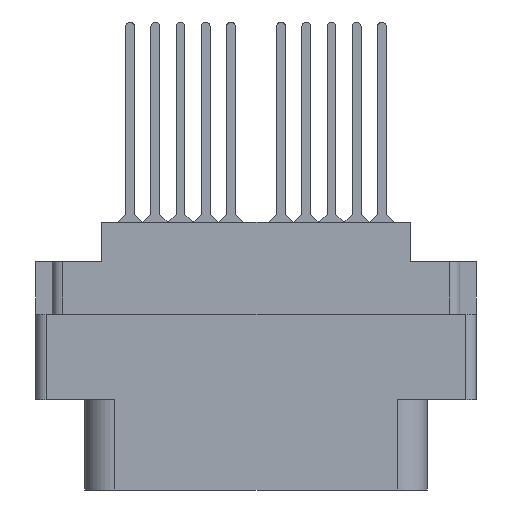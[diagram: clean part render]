
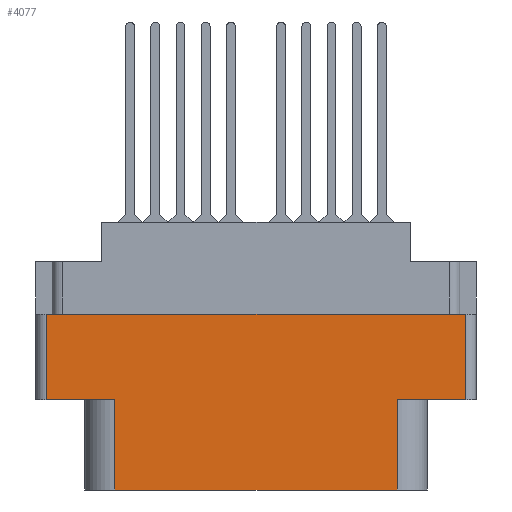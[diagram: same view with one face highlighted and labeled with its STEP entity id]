
A CAD part, front view. The second image highlights one B-rep face of the part: STEP entity #4077.
In plain terms, the highlighted planar face has unit normal (0, -1, 0).
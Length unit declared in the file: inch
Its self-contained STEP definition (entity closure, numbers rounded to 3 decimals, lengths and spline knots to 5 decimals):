
#502 = VECTOR ( 'NONE', #12374, 39.37008 ) ;
#558 = FACE_OUTER_BOUND ( 'NONE', #7926, .T. ) ;
#687 = VERTEX_POINT ( 'NONE', #7969 ) ;
#767 = CARTESIAN_POINT ( 'NONE',  ( -0.42052, -0.343, -0.798 ) ) ;
#2515 = VECTOR ( 'NONE', #4962, 39.37008 ) ;
#2782 = VERTEX_POINT ( 'NONE', #19760 ) ;
#3194 = ORIENTED_EDGE ( 'NONE', *, *, #14946, .T. ) ;
#4077 = ADVANCED_FACE ( 'NONE', ( #558 ), #27194, .T. ) ;
#4551 = VECTOR ( 'NONE', #13464, 39.37008 ) ;
#4962 = DIRECTION ( 'NONE',  ( 0., 0., -1. ) ) ;
#5088 = VECTOR ( 'NONE', #18477, 39.37008 ) ;
#5270 = DIRECTION ( 'NONE',  ( -1., 0., 0. ) ) ;
#5711 = CARTESIAN_POINT ( 'NONE',  ( 0.624, -0.343, -0.529 ) ) ;
#5946 = EDGE_CURVE ( 'NONE', #23747, #13217, #25041, .T. ) ;
#6018 = CARTESIAN_POINT ( 'NONE',  ( 0.624, -0.343, -0.274 ) ) ;
#6311 = ORIENTED_EDGE ( 'NONE', *, *, #12337, .T. ) ;
#6898 = CARTESIAN_POINT ( 'NONE',  ( -0.42052, -0.343, -0.529 ) ) ;
#7129 = LINE ( 'NONE', #11710, #5088 ) ;
#7200 = LINE ( 'NONE', #22389, #12022 ) ;
#7605 = AXIS2_PLACEMENT_3D ( 'NONE', #9855, #12155, #18536 ) ;
#7799 = ORIENTED_EDGE ( 'NONE', *, *, #14473, .F. ) ;
#7926 = EDGE_LOOP ( 'NONE', ( #25615, #3194, #23369, #15435, #6311, #18955, #7799, #14223 ) ) ;
#7969 = CARTESIAN_POINT ( 'NONE',  ( -0.42052, -0.343, -0.798 ) ) ;
#9855 = CARTESIAN_POINT ( 'NONE',  ( -0.656, -0.343, -0.798 ) ) ;
#10859 = DIRECTION ( 'NONE',  ( 0., 0., 1. ) ) ;
#11710 = CARTESIAN_POINT ( 'NONE',  ( 0., -0.343, -0.274 ) ) ;
#11861 = DIRECTION ( 'NONE',  ( 0., 0., -1. ) ) ;
#12022 = VECTOR ( 'NONE', #5270, 39.37008 ) ;
#12155 = DIRECTION ( 'NONE',  ( 0., -1., 0. ) ) ;
#12337 = EDGE_CURVE ( 'NONE', #687, #16984, #18858, .T. ) ;
#12374 = DIRECTION ( 'NONE',  ( 0., 0., 1. ) ) ;
#12659 = CARTESIAN_POINT ( 'NONE',  ( 0.42052, -0.343, -0.529 ) ) ;
#13217 = VERTEX_POINT ( 'NONE', #6898 ) ;
#13447 = VERTEX_POINT ( 'NONE', #23145 ) ;
#13464 = DIRECTION ( 'NONE',  ( 1., 0., 0. ) ) ;
#13751 = VECTOR ( 'NONE', #26379, 39.37008 ) ;
#14223 = ORIENTED_EDGE ( 'NONE', *, *, #26469, .T. ) ;
#14473 = EDGE_CURVE ( 'NONE', #23448, #13447, #7200, .T. ) ;
#14946 = EDGE_CURVE ( 'NONE', #2782, #23747, #23919, .T. ) ;
#15219 = VECTOR ( 'NONE', #10859, 39.37008 ) ;
#15435 = ORIENTED_EDGE ( 'NONE', *, *, #22451, .T. ) ;
#15484 = CARTESIAN_POINT ( 'NONE',  ( 0., -0.343, -0.529 ) ) ;
#15958 = EDGE_CURVE ( 'NONE', #2782, #24974, #7129, .T. ) ;
#16259 = CARTESIAN_POINT ( 'NONE',  ( -0.624, -0.343, -0.798 ) ) ;
#16984 = VERTEX_POINT ( 'NONE', #24379 ) ;
#18477 = DIRECTION ( 'NONE',  ( 1., 0., 0. ) ) ;
#18536 = DIRECTION ( 'NONE',  ( 0., 0., -1. ) ) ;
#18858 = LINE ( 'NONE', #20015, #13751 ) ;
#18955 = ORIENTED_EDGE ( 'NONE', *, *, #19255, .T. ) ;
#18972 = LINE ( 'NONE', #12659, #502 ) ;
#19255 = EDGE_CURVE ( 'NONE', #16984, #13447, #18972, .T. ) ;
#19551 = CARTESIAN_POINT ( 'NONE',  ( -0.624, -0.343, -0.529 ) ) ;
#19760 = CARTESIAN_POINT ( 'NONE',  ( -0.624, -0.343, -0.274 ) ) ;
#20015 = CARTESIAN_POINT ( 'NONE',  ( -0.656, -0.343, -0.798 ) ) ;
#20329 = LINE ( 'NONE', #26192, #15219 ) ;
#20849 = LINE ( 'NONE', #767, #2515 ) ;
#22389 = CARTESIAN_POINT ( 'NONE',  ( 0., -0.343, -0.529 ) ) ;
#22451 = EDGE_CURVE ( 'NONE', #13217, #687, #20849, .T. ) ;
#23145 = CARTESIAN_POINT ( 'NONE',  ( 0.42052, -0.343, -0.529 ) ) ;
#23369 = ORIENTED_EDGE ( 'NONE', *, *, #5946, .T. ) ;
#23448 = VERTEX_POINT ( 'NONE', #5711 ) ;
#23747 = VERTEX_POINT ( 'NONE', #19551 ) ;
#23919 = LINE ( 'NONE', #16259, #27991 ) ;
#24379 = CARTESIAN_POINT ( 'NONE',  ( 0.42052, -0.343, -0.798 ) ) ;
#24974 = VERTEX_POINT ( 'NONE', #6018 ) ;
#25041 = LINE ( 'NONE', #15484, #4551 ) ;
#25615 = ORIENTED_EDGE ( 'NONE', *, *, #15958, .F. ) ;
#26192 = CARTESIAN_POINT ( 'NONE',  ( 0.624, -0.343, -0.798 ) ) ;
#26379 = DIRECTION ( 'NONE',  ( 1., 0., 0. ) ) ;
#26469 = EDGE_CURVE ( 'NONE', #23448, #24974, #20329, .T. ) ;
#27194 = PLANE ( 'NONE',  #7605 ) ;
#27991 = VECTOR ( 'NONE', #11861, 39.37008 ) ;
